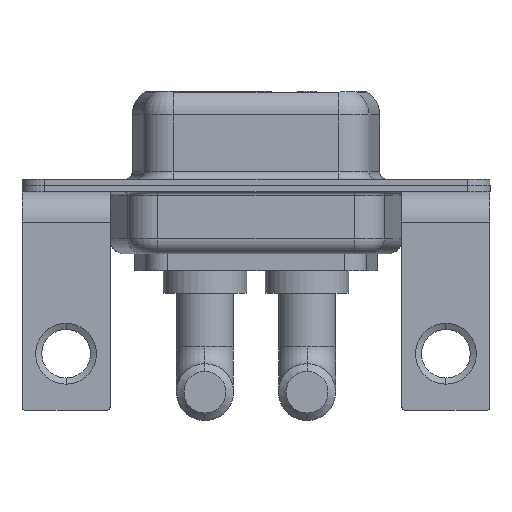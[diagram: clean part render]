
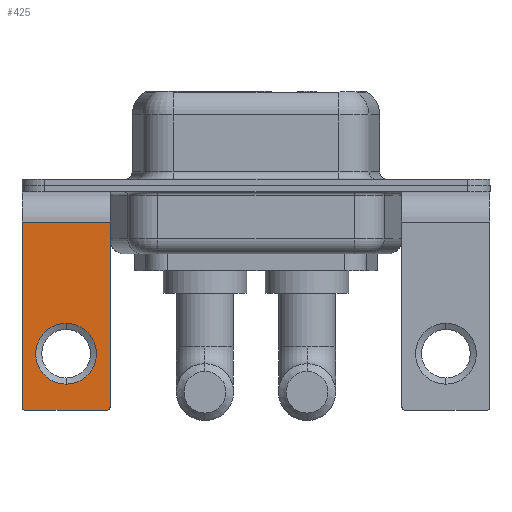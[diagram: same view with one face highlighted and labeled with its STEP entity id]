
A CAD part, front view. The second image highlights one B-rep face of the part: STEP entity #425.
In plain terms, the highlighted planar face has unit normal (0, -1, 0).
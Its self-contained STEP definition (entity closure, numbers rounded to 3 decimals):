
#280 = DIRECTION ( 'NONE',  ( -1., 0., 0. ) ) ;
#425 = ADVANCED_FACE ( 'NONE', ( #5018, #3959 ), #9372, .F. ) ;
#531 = EDGE_LOOP ( 'NONE', ( #6039, #13023 ) ) ;
#552 = ORIENTED_EDGE ( 'NONE', *, *, #3242, .T. ) ;
#709 = CARTESIAN_POINT ( 'NONE',  ( -2.65, -6.25, -14.8 ) ) ;
#810 = DIRECTION ( 'NONE',  ( 0., 0., -1. ) ) ;
#992 = CARTESIAN_POINT ( 'NONE',  ( -2.9, -6.25, -14.55 ) ) ;
#1104 = ORIENTED_EDGE ( 'NONE', *, *, #13929, .T. ) ;
#1337 = CARTESIAN_POINT ( 'NONE',  ( 0., -6.25, -11.07 ) ) ;
#1953 = CARTESIAN_POINT ( 'NONE',  ( 0., -6.25, -11.07 ) ) ;
#2006 = CIRCLE ( 'NONE', #9973, 0.25 ) ;
#2325 = EDGE_CURVE ( 'NONE', #5174, #10176, #8962, .T. ) ;
#2432 = DIRECTION ( 'NONE',  ( 0., -1., 0. ) ) ;
#2602 = VERTEX_POINT ( 'NONE', #709 ) ;
#2746 = CARTESIAN_POINT ( 'NONE',  ( -2.65, -6.25, -14.55 ) ) ;
#3084 = VECTOR ( 'NONE', #11953, 1000. ) ;
#3103 = DIRECTION ( 'NONE',  ( 0., 0., 1. ) ) ;
#3242 = EDGE_CURVE ( 'NONE', #12250, #10287, #12955, .T. ) ;
#3695 = LINE ( 'NONE', #12385, #3953 ) ;
#3698 = CARTESIAN_POINT ( 'NONE',  ( 0., -6.25, -9.07 ) ) ;
#3953 = VECTOR ( 'NONE', #6969, 1000. ) ;
#3959 = FACE_OUTER_BOUND ( 'NONE', #13906, .T. ) ;
#4239 = EDGE_CURVE ( 'NONE', #4663, #8445, #5782, .T. ) ;
#4659 = VECTOR ( 'NONE', #810, 1000. ) ;
#4663 = VERTEX_POINT ( 'NONE', #5608 ) ;
#4681 = EDGE_CURVE ( 'NONE', #10176, #5174, #5531, .T. ) ;
#4978 = VERTEX_POINT ( 'NONE', #992 ) ;
#5018 = FACE_BOUND ( 'NONE', #531, .T. ) ;
#5174 = VERTEX_POINT ( 'NONE', #3698 ) ;
#5460 = CARTESIAN_POINT ( 'NONE',  ( 2.9, -6.25, -2.4 ) ) ;
#5531 = CIRCLE ( 'NONE', #10998, 2. ) ;
#5608 = CARTESIAN_POINT ( 'NONE',  ( 2.65, -6.25, -14.8 ) ) ;
#5637 = DIRECTION ( 'NONE',  ( 0., 0., 1. ) ) ;
#5672 = DIRECTION ( 'NONE',  ( 0., 1., 0. ) ) ;
#5782 = CIRCLE ( 'NONE', #11257, 0.25 ) ;
#6039 = ORIENTED_EDGE ( 'NONE', *, *, #4681, .T. ) ;
#6063 = CARTESIAN_POINT ( 'NONE',  ( 2.9, -6.25, -2.4 ) ) ;
#6173 = ORIENTED_EDGE ( 'NONE', *, *, #8278, .F. ) ;
#6369 = ORIENTED_EDGE ( 'NONE', *, *, #11163, .T. ) ;
#6969 = DIRECTION ( 'NONE',  ( 0., 0., -1. ) ) ;
#7087 = CARTESIAN_POINT ( 'NONE',  ( 2.9, -6.25, -2.4 ) ) ;
#8278 = EDGE_CURVE ( 'NONE', #12250, #8445, #12782, .T. ) ;
#8445 = VERTEX_POINT ( 'NONE', #13214 ) ;
#8502 = AXIS2_PLACEMENT_3D ( 'NONE', #1953, #9641, #3103 ) ;
#8713 = DIRECTION ( 'NONE',  ( 0., 0., 1. ) ) ;
#8761 = ORIENTED_EDGE ( 'NONE', *, *, #12572, .F. ) ;
#8962 = CIRCLE ( 'NONE', #8502, 2. ) ;
#9372 = PLANE ( 'NONE',  #11532 ) ;
#9411 = CARTESIAN_POINT ( 'NONE',  ( 0., -6.25, -13.07 ) ) ;
#9641 = DIRECTION ( 'NONE',  ( 0., 1., 0. ) ) ;
#9803 = ORIENTED_EDGE ( 'NONE', *, *, #4239, .T. ) ;
#9973 = AXIS2_PLACEMENT_3D ( 'NONE', #2746, #10368, #12789 ) ;
#10176 = VERTEX_POINT ( 'NONE', #9411 ) ;
#10287 = VERTEX_POINT ( 'NONE', #10911 ) ;
#10368 = DIRECTION ( 'NONE',  ( 0., -1., 0. ) ) ;
#10911 = CARTESIAN_POINT ( 'NONE',  ( -2.9, -6.25, -2.4 ) ) ;
#10998 = AXIS2_PLACEMENT_3D ( 'NONE', #1337, #5672, #11230 ) ;
#11163 = EDGE_CURVE ( 'NONE', #4978, #2602, #2006, .T. ) ;
#11230 = DIRECTION ( 'NONE',  ( 0., 0., 1. ) ) ;
#11248 = CARTESIAN_POINT ( 'NONE',  ( 2.9, -6.25, -14.8 ) ) ;
#11257 = AXIS2_PLACEMENT_3D ( 'NONE', #12196, #2432, #5637 ) ;
#11445 = DIRECTION ( 'NONE',  ( 0., 1., 0. ) ) ;
#11532 = AXIS2_PLACEMENT_3D ( 'NONE', #7087, #11445, #8713 ) ;
#11953 = DIRECTION ( 'NONE',  ( -1., 0., 0. ) ) ;
#12196 = CARTESIAN_POINT ( 'NONE',  ( 2.65, -6.25, -14.55 ) ) ;
#12250 = VERTEX_POINT ( 'NONE', #6063 ) ;
#12385 = CARTESIAN_POINT ( 'NONE',  ( -2.9, -6.25, -2.4 ) ) ;
#12572 = EDGE_CURVE ( 'NONE', #4663, #2602, #13540, .T. ) ;
#12720 = CARTESIAN_POINT ( 'NONE',  ( 2.9, -6.25, -2.4 ) ) ;
#12782 = LINE ( 'NONE', #12720, #4659 ) ;
#12789 = DIRECTION ( 'NONE',  ( 0., 0., 1. ) ) ;
#12955 = LINE ( 'NONE', #5460, #3084 ) ;
#13023 = ORIENTED_EDGE ( 'NONE', *, *, #2325, .T. ) ;
#13038 = VECTOR ( 'NONE', #280, 1000. ) ;
#13214 = CARTESIAN_POINT ( 'NONE',  ( 2.9, -6.25, -14.55 ) ) ;
#13540 = LINE ( 'NONE', #11248, #13038 ) ;
#13906 = EDGE_LOOP ( 'NONE', ( #1104, #6369, #8761, #9803, #6173, #552 ) ) ;
#13929 = EDGE_CURVE ( 'NONE', #10287, #4978, #3695, .T. ) ;
